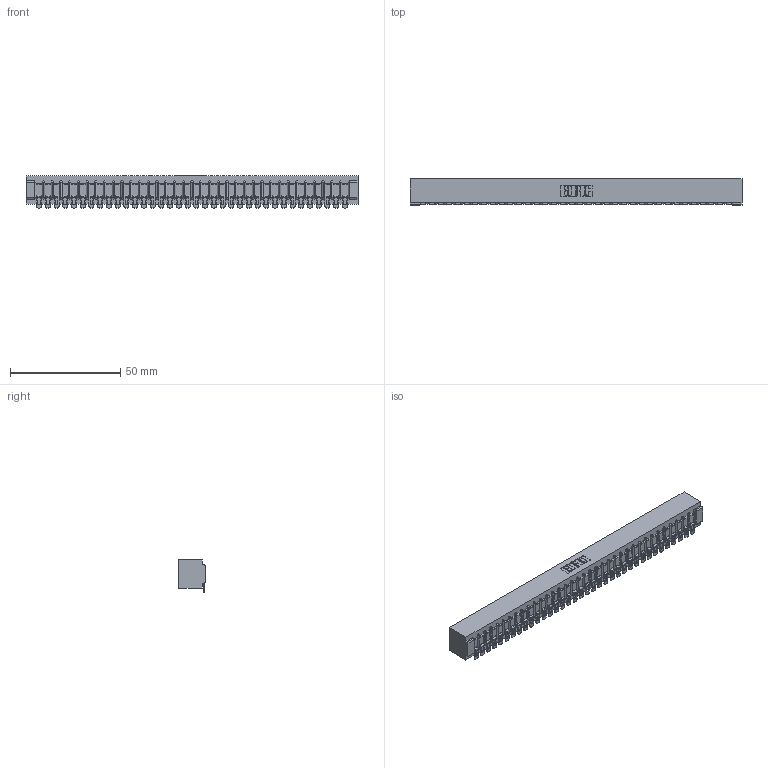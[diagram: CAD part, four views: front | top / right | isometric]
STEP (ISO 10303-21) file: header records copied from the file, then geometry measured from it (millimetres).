
FILE_DESCRIPTION (( 'STEP AP203' ), '1' );
FILE_NAME ('357-036-454-101.STEP', '2020-10-02T17:42:27', ( '' ), ( '' ), 'SwSTEP 2.0', 'SolidWorks 2020', '' );
FILE_SCHEMA (( 'CONFIG_CONTROL_DESIGN' ));
Length unit declared in the file: inch
Products named in the file (3): 307 Part_No Mounting Lugs; 307-290-002_554; 357-036-454-101
Assembly tree (37 placements, depth 2):
  357-036-454-101
    307 Part_No Mounting Lugs
    307-290-002_554  x36
Bounding box: 150.52 x 12.01 x 14.52 mm (x, y, z)
Volume: 16633.6 mm3; surface area: 21271.2 mm2
Topology: 37 solids, 37 shells, 3063 faces, 9407 edges, 6170 vertices
Faces by surface type: plane 1722, cylinder 1267, sphere 74
Entity records: 32289 total; most frequent: CARTESIAN_POINT 5446, ORIENTED_EDGE 5436, DIRECTION 5298, EDGE_CURVE 2718, LINE 2074, VECTOR 2074, VERTEX_POINT 1760, AXIS2_PLACEMENT_3D 1612
